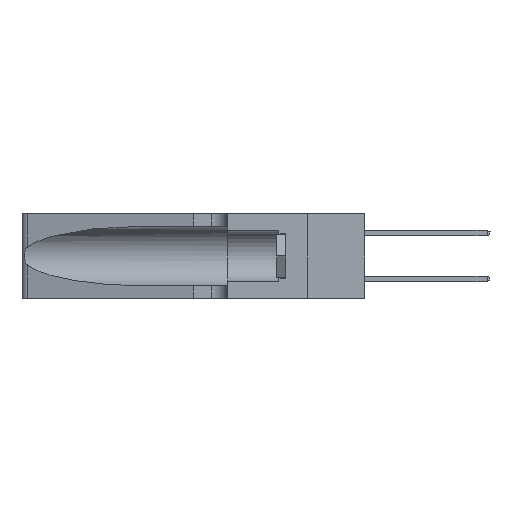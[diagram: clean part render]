
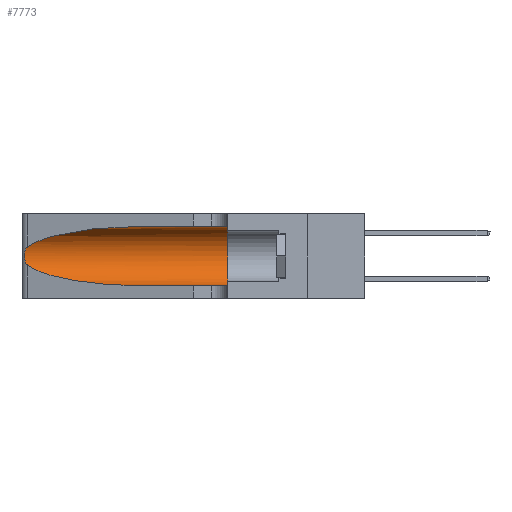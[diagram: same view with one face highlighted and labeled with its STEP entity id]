
A CAD part, left-side view. The second image highlights one B-rep face of the part: STEP entity #7773.
In plain terms, the highlighted cylindrical face has radius 3.308 mm (diameter 6.617 mm), a partial arc.
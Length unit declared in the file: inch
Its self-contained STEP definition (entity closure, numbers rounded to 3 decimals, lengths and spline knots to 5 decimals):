
#977 = CARTESIAN_POINT ( 'NONE',  ( 0.26017, 1.23833, 0.17102 ) ) ;
#1136 = CARTESIAN_POINT ( 'NONE',  ( 0.25639, 1.23186, 0.15144 ) ) ;
#1185 = CARTESIAN_POINT ( 'NONE',  ( 0.1305, 1.61858, 0.185 ) ) ;
#1453 = CARTESIAN_POINT ( 'NONE',  ( 0.26075, 1.23896, 0.19203 ) ) ;
#2034 = CIRCLE ( 'NONE', #19383, 0.13025 ) ;
#2160 = CARTESIAN_POINT ( 'NONE',  ( 0.2373, 1.15595, 0.08982 ) ) ;
#5044 = CARTESIAN_POINT ( 'NONE',  ( 0.25555, 1.22994, 0.2215 ) ) ;
#5860 = CARTESIAN_POINT ( 'NONE',  ( 0.25487, 1.22718, 0.22369 ) ) ;
#6004 = CARTESIAN_POINT ( 'NONE',  ( 0.1305, 0.72297, 0.31525 ) ) ;
#6300 = DIRECTION ( 'NONE',  ( 0., -1., 0. ) ) ;
#6352 =( BOUNDED_CURVE ( )  B_SPLINE_CURVE ( 3, ( #19652, #2160, #23384, #38203 ),
 .UNSPECIFIED., .F., .T. ) 
 B_SPLINE_CURVE_WITH_KNOTS ( ( 4, 4 ),
 ( 3.44316, 4.71239 ),
 .UNSPECIFIED. ) 
 CURVE ( )  GEOMETRIC_REPRESENTATION_ITEM ( )  RATIONAL_B_SPLINE_CURVE ( ( 1., 0.87, 0.87, 1. ) ) 
 REPRESENTATION_ITEM ( '' )  );
#6812 = CARTESIAN_POINT ( 'NONE',  ( 0.1305, 0.72297, 0.05475 ) ) ;
#7773 = ADVANCED_FACE ( 'NONE', ( #23764 ), #15420, .F. ) ;
#7861 = EDGE_CURVE ( 'NONE', #29200, #41653, #35519, .T. ) ;
#8337 = CARTESIAN_POINT ( 'NONE',  ( 0.25487, 1.22718, 0.14631 ) ) ;
#9746 = CARTESIAN_POINT ( 'NONE',  ( 0.25487, 1.22718, 0.14631 ) ) ;
#10157 = ORIENTED_EDGE ( 'NONE', *, *, #33111, .T. ) ;
#14744 = VERTEX_POINT ( 'NONE', #9746 ) ;
#15204 = CARTESIAN_POINT ( 'NONE',  ( 0.25639, 1.23184, 0.21858 ) ) ;
#15420 = CYLINDRICAL_SURFACE ( 'NONE', #24602, 0.13025 ) ;
#15503 = B_SPLINE_CURVE_WITH_KNOTS ( 'NONE', 3,
 ( #36899, #5044, #15204, #29859, #43731, #19247, #1453, #26419, #977, #30005, #25975, #1136, #29686, #8337 ),
 .UNSPECIFIED., .F., .F.,
 ( 4, 2, 2, 2, 2, 2, 4 ),
 ( 0., 0.00027, 0.00053, 0.00107, 0.0016, 0.00187, 0.00214 ),
 .UNSPECIFIED. ) ;
#15555 = DIRECTION ( 'NONE',  ( 0., -1., 0. ) ) ;
#17321 = LINE ( 'NONE', #31553, #27932 ) ;
#17470 = DIRECTION ( 'NONE',  ( 0., -1., 0. ) ) ;
#19247 = CARTESIAN_POINT ( 'NONE',  ( 0.26018, 1.23835, 0.19895 ) ) ;
#19383 = AXIS2_PLACEMENT_3D ( 'NONE', #27866, #38651, #23674 ) ;
#19652 = CARTESIAN_POINT ( 'NONE',  ( 0.25487, 1.22718, 0.14631 ) ) ;
#20031 = CARTESIAN_POINT ( 'NONE',  ( 0.18966, 0.96281, 0.31525 ) ) ;
#21093 = ORIENTED_EDGE ( 'NONE', *, *, #7861, .T. ) ;
#22278 = VERTEX_POINT ( 'NONE', #30545 ) ;
#23384 = CARTESIAN_POINT ( 'NONE',  ( 0.18966, 0.96281, 0.05475 ) ) ;
#23674 = DIRECTION ( 'NONE',  ( 0., 0., 1. ) ) ;
#23726 = CARTESIAN_POINT ( 'NONE',  ( 0.1305, 1.61858, 0.05475 ) ) ;
#23764 = FACE_OUTER_BOUND ( 'NONE', #45641, .T. ) ;
#24260 = EDGE_CURVE ( 'NONE', #14744, #37493, #6352, .T. ) ;
#24602 = AXIS2_PLACEMENT_3D ( 'NONE', #1185, #15555, #44239 ) ;
#25975 = CARTESIAN_POINT ( 'NONE',  ( 0.25789, 1.23486, 0.15765 ) ) ;
#26419 = CARTESIAN_POINT ( 'NONE',  ( 0.26075, 1.23896, 0.178 ) ) ;
#26444 = EDGE_CURVE ( 'NONE', #38350, #22278, #2034, .T. ) ;
#27866 = CARTESIAN_POINT ( 'NONE',  ( 0.1305, 0.35, 0.185 ) ) ;
#27932 = VECTOR ( 'NONE', #6300, 39.37008 ) ;
#27997 = ORIENTED_EDGE ( 'NONE', *, *, #38404, .T. ) ;
#29200 = VERTEX_POINT ( 'NONE', #29367 ) ;
#29366 = CARTESIAN_POINT ( 'NONE',  ( 0.25487, 1.22718, 0.22369 ) ) ;
#29367 = CARTESIAN_POINT ( 'NONE',  ( 0.1305, 0.72297, 0.31525 ) ) ;
#29686 = CARTESIAN_POINT ( 'NONE',  ( 0.25555, 1.22993, 0.14849 ) ) ;
#29859 = CARTESIAN_POINT ( 'NONE',  ( 0.25787, 1.23484, 0.2124 ) ) ;
#30005 = CARTESIAN_POINT ( 'NONE',  ( 0.25856, 1.23593, 0.16098 ) ) ;
#30545 = CARTESIAN_POINT ( 'NONE',  ( 0.1305, 0.35, 0.05475 ) ) ;
#31553 = CARTESIAN_POINT ( 'NONE',  ( 0.1305, 1.61858, 0.31525 ) ) ;
#33111 = EDGE_CURVE ( 'NONE', #37493, #22278, #40516, .T. ) ;
#35519 =( BOUNDED_CURVE ( )  B_SPLINE_CURVE ( 3, ( #6004, #20031, #38148, #5860 ),
 .UNSPECIFIED., .F., .F. ) 
 B_SPLINE_CURVE_WITH_KNOTS ( ( 4, 4 ),
 ( 1.5708, 2.84003 ),
 .UNSPECIFIED. ) 
 CURVE ( )  GEOMETRIC_REPRESENTATION_ITEM ( )  RATIONAL_B_SPLINE_CURVE ( ( 1., 0.87, 0.87, 1. ) ) 
 REPRESENTATION_ITEM ( '' )  );
#36899 = CARTESIAN_POINT ( 'NONE',  ( 0.25487, 1.22718, 0.22369 ) ) ;
#37493 = VERTEX_POINT ( 'NONE', #6812 ) ;
#38148 = CARTESIAN_POINT ( 'NONE',  ( 0.2373, 1.15595, 0.28018 ) ) ;
#38203 = CARTESIAN_POINT ( 'NONE',  ( 0.1305, 0.72297, 0.05475 ) ) ;
#38350 = VERTEX_POINT ( 'NONE', #44039 ) ;
#38404 = EDGE_CURVE ( 'NONE', #41653, #14744, #15503, .T. ) ;
#38651 = DIRECTION ( 'NONE',  ( 0., 1., 0. ) ) ;
#39491 = EDGE_CURVE ( 'NONE', #29200, #38350, #17321, .T. ) ;
#39811 = ORIENTED_EDGE ( 'NONE', *, *, #39491, .F. ) ;
#39922 = VECTOR ( 'NONE', #17470, 39.37008 ) ;
#40516 = LINE ( 'NONE', #23726, #39922 ) ;
#41653 = VERTEX_POINT ( 'NONE', #29366 ) ;
#43683 = ORIENTED_EDGE ( 'NONE', *, *, #24260, .T. ) ;
#43731 = CARTESIAN_POINT ( 'NONE',  ( 0.25854, 1.2359, 0.20912 ) ) ;
#44039 = CARTESIAN_POINT ( 'NONE',  ( 0.1305, 0.35, 0.31525 ) ) ;
#44239 = DIRECTION ( 'NONE',  ( 0., 0., -1. ) ) ;
#44634 = ORIENTED_EDGE ( 'NONE', *, *, #26444, .F. ) ;
#45641 = EDGE_LOOP ( 'NONE', ( #21093, #27997, #43683, #10157, #44634, #39811 ) ) ;
